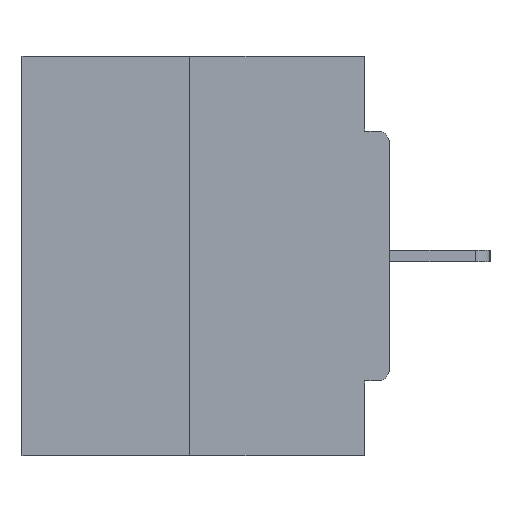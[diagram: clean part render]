
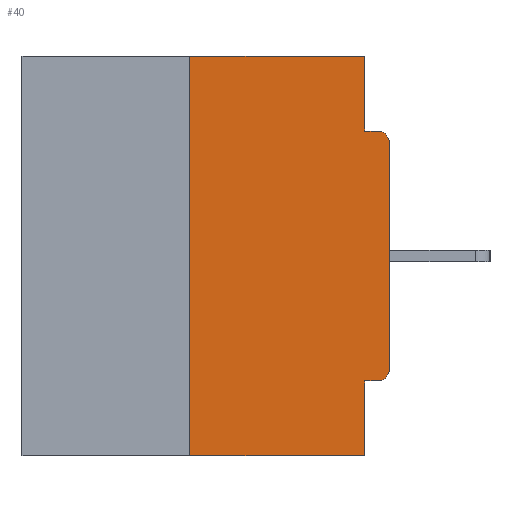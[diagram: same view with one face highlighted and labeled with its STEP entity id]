
A CAD part, left-side view. The second image highlights one B-rep face of the part: STEP entity #40.
In plain terms, the highlighted planar face has unit normal (-1, 0, 0).
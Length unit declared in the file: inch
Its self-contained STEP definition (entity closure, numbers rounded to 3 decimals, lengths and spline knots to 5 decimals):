
#40 = ADVANCED_FACE ( 'NONE', ( #22499 ), #15782, .F. ) ;
#205 = VERTEX_POINT ( 'NONE', #11380 ) ;
#589 = ORIENTED_EDGE ( 'NONE', *, *, #6843, .T. ) ;
#1489 = DIRECTION ( 'NONE',  ( 0., -1., 0. ) ) ;
#1624 = CARTESIAN_POINT ( 'NONE',  ( 0., 0.015, -0.3915 ) ) ;
#2088 = CARTESIAN_POINT ( 'NONE',  ( 0., 0.25, 0. ) ) ;
#2198 = VECTOR ( 'NONE', #28497, 39.37008 ) ;
#2488 = CARTESIAN_POINT ( 'NONE',  ( 0., 0.25, -0.5 ) ) ;
#2971 = CARTESIAN_POINT ( 'NONE',  ( 0., 0., 0. ) ) ;
#3547 = EDGE_CURVE ( 'NONE', #8241, #27307, #22784, .T. ) ;
#3557 = AXIS2_PLACEMENT_3D ( 'NONE', #1624, #26004, #10292 ) ;
#3618 = VECTOR ( 'NONE', #1489, 39.37008 ) ;
#3654 = CARTESIAN_POINT ( 'NONE',  ( 0., 0.031, 0. ) ) ;
#4170 = EDGE_CURVE ( 'NONE', #22276, #28082, #18328, .T. ) ;
#5634 = DIRECTION ( 'NONE',  ( 0., 0., 1. ) ) ;
#5927 = VECTOR ( 'NONE', #26572, 39.37008 ) ;
#5993 = ORIENTED_EDGE ( 'NONE', *, *, #28563, .F. ) ;
#6843 = EDGE_CURVE ( 'NONE', #14662, #23718, #26204, .T. ) ;
#7085 = EDGE_CURVE ( 'NONE', #205, #26147, #11058, .T. ) ;
#7207 = DIRECTION ( 'NONE',  ( 1., 0., 0. ) ) ;
#7309 = EDGE_CURVE ( 'NONE', #16314, #16543, #19620, .T. ) ;
#7715 = EDGE_LOOP ( 'NONE', ( #15884, #13817, #589, #24111, #16234, #12972, #21546, #10961, #27614, #5993 ) ) ;
#8241 = VERTEX_POINT ( 'NONE', #2088 ) ;
#8322 = CARTESIAN_POINT ( 'NONE',  ( 0., 0.015, -0.1085 ) ) ;
#8789 = VECTOR ( 'NONE', #5634, 39.37008 ) ;
#8891 = CARTESIAN_POINT ( 'NONE',  ( 0., 0., -0.4065 ) ) ;
#10292 = DIRECTION ( 'NONE',  ( 0., 0., -1. ) ) ;
#10736 = DIRECTION ( 'NONE',  ( 0., 0., -1. ) ) ;
#10790 = VECTOR ( 'NONE', #25333, 39.37008 ) ;
#10961 = ORIENTED_EDGE ( 'NONE', *, *, #25891, .T. ) ;
#11030 = LINE ( 'NONE', #17286, #5927 ) ;
#11058 = LINE ( 'NONE', #8891, #17051 ) ;
#11380 = CARTESIAN_POINT ( 'NONE',  ( 0., 0.015, -0.4065 ) ) ;
#11729 = CARTESIAN_POINT ( 'NONE',  ( 0., 0.031, -0.0935 ) ) ;
#12303 = CARTESIAN_POINT ( 'NONE',  ( 0., 0.25, 0. ) ) ;
#12501 = CARTESIAN_POINT ( 'NONE',  ( 0., 0., -0.0935 ) ) ;
#12972 = ORIENTED_EDGE ( 'NONE', *, *, #27280, .T. ) ;
#13817 = ORIENTED_EDGE ( 'NONE', *, *, #16530, .F. ) ;
#13893 = DIRECTION ( 'NONE',  ( 0., -1., 0. ) ) ;
#14341 = CARTESIAN_POINT ( 'NONE',  ( 0., 0.015, -0.0935 ) ) ;
#14442 = AXIS2_PLACEMENT_3D ( 'NONE', #20279, #7207, #17956 ) ;
#14662 = VERTEX_POINT ( 'NONE', #2488 ) ;
#15782 = PLANE ( 'NONE',  #14442 ) ;
#15884 = ORIENTED_EDGE ( 'NONE', *, *, #3547, .F. ) ;
#16151 = AXIS2_PLACEMENT_3D ( 'NONE', #8322, #21722, #19323 ) ;
#16234 = ORIENTED_EDGE ( 'NONE', *, *, #7085, .F. ) ;
#16314 = VERTEX_POINT ( 'NONE', #11729 ) ;
#16530 = EDGE_CURVE ( 'NONE', #14662, #8241, #16932, .T. ) ;
#16543 = VERTEX_POINT ( 'NONE', #14341 ) ;
#16932 = LINE ( 'NONE', #12303, #8789 ) ;
#17051 = VECTOR ( 'NONE', #20337, 39.37008 ) ;
#17286 = CARTESIAN_POINT ( 'NONE',  ( 0., 0.031, -0.5 ) ) ;
#17457 = CIRCLE ( 'NONE', #3557, 0.015 ) ;
#17956 = DIRECTION ( 'NONE',  ( 0., 0., -1. ) ) ;
#18328 = LINE ( 'NONE', #2971, #10790 ) ;
#18405 = VECTOR ( 'NONE', #10736, 39.37008 ) ;
#18519 = CARTESIAN_POINT ( 'NONE',  ( 0., 0.46, 0. ) ) ;
#18613 = VECTOR ( 'NONE', #13893, 39.37008 ) ;
#19169 = CARTESIAN_POINT ( 'NONE',  ( 0., 0.031, 0. ) ) ;
#19322 = LINE ( 'NONE', #19169, #18405 ) ;
#19323 = DIRECTION ( 'NONE',  ( 0., 0., -1. ) ) ;
#19620 = LINE ( 'NONE', #12501, #3618 ) ;
#20279 = CARTESIAN_POINT ( 'NONE',  ( 0., 0.46, 0. ) ) ;
#20302 = CIRCLE ( 'NONE', #16151, 0.015 ) ;
#20337 = DIRECTION ( 'NONE',  ( 0., 1., 0. ) ) ;
#21506 = CARTESIAN_POINT ( 'NONE',  ( 0., 0.031, -0.4065 ) ) ;
#21546 = ORIENTED_EDGE ( 'NONE', *, *, #4170, .T. ) ;
#21722 = DIRECTION ( 'NONE',  ( -1., 0., 0. ) ) ;
#22208 = CARTESIAN_POINT ( 'NONE',  ( 0., 0.031, -0.5 ) ) ;
#22276 = VERTEX_POINT ( 'NONE', #23237 ) ;
#22499 = FACE_OUTER_BOUND ( 'NONE', #7715, .T. ) ;
#22784 = LINE ( 'NONE', #18519, #18613 ) ;
#23237 = CARTESIAN_POINT ( 'NONE',  ( 0., 0., -0.3915 ) ) ;
#23268 = EDGE_CURVE ( 'NONE', #26147, #23718, #11030, .T. ) ;
#23718 = VERTEX_POINT ( 'NONE', #22208 ) ;
#24111 = ORIENTED_EDGE ( 'NONE', *, *, #23268, .F. ) ;
#25333 = DIRECTION ( 'NONE',  ( 0., 0., 1. ) ) ;
#25891 = EDGE_CURVE ( 'NONE', #28082, #16543, #20302, .T. ) ;
#26004 = DIRECTION ( 'NONE',  ( -1., 0., 0. ) ) ;
#26147 = VERTEX_POINT ( 'NONE', #21506 ) ;
#26204 = LINE ( 'NONE', #27913, #2198 ) ;
#26467 = CARTESIAN_POINT ( 'NONE',  ( 0., 0., -0.1085 ) ) ;
#26572 = DIRECTION ( 'NONE',  ( 0., 0., -1. ) ) ;
#27280 = EDGE_CURVE ( 'NONE', #205, #22276, #17457, .T. ) ;
#27307 = VERTEX_POINT ( 'NONE', #3654 ) ;
#27614 = ORIENTED_EDGE ( 'NONE', *, *, #7309, .F. ) ;
#27913 = CARTESIAN_POINT ( 'NONE',  ( 0., 0.46, -0.5 ) ) ;
#28082 = VERTEX_POINT ( 'NONE', #26467 ) ;
#28497 = DIRECTION ( 'NONE',  ( 0., -1., 0. ) ) ;
#28563 = EDGE_CURVE ( 'NONE', #27307, #16314, #19322, .T. ) ;
